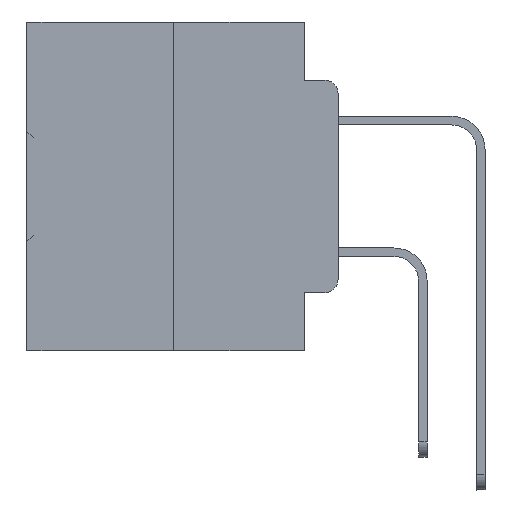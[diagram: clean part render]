
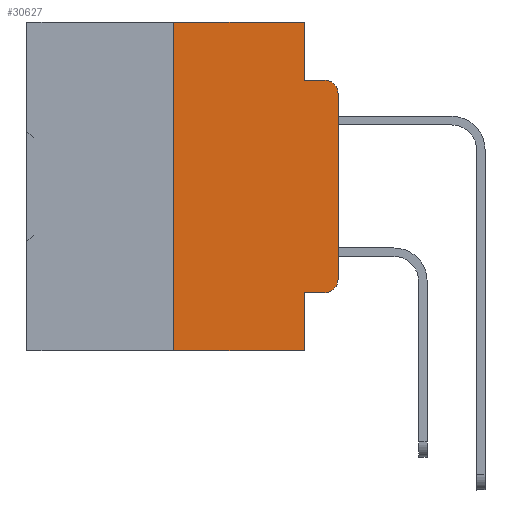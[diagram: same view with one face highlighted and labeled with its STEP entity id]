
A CAD part, left-side view. The second image highlights one B-rep face of the part: STEP entity #30627.
In plain terms, the highlighted planar face has unit normal (-1, 0, 0).
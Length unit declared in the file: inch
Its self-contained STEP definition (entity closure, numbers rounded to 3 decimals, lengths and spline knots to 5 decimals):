
#552 = CARTESIAN_POINT ( 'NONE',  ( 0., 0.25, 0. ) ) ;
#585 = DIRECTION ( 'NONE',  ( 0., 0., -1. ) ) ;
#738 = EDGE_CURVE ( 'NONE', #4777, #22115, #18678, .T. ) ;
#2525 = ORIENTED_EDGE ( 'NONE', *, *, #8999, .T. ) ;
#2659 = VERTEX_POINT ( 'NONE', #24589 ) ;
#2693 = VERTEX_POINT ( 'NONE', #31869 ) ;
#3128 = CARTESIAN_POINT ( 'NONE',  ( 0., 0.051, -0.4115 ) ) ;
#4285 = VERTEX_POINT ( 'NONE', #552 ) ;
#4529 = CARTESIAN_POINT ( 'NONE',  ( 0., 0.051, -0.4115 ) ) ;
#4596 = VECTOR ( 'NONE', #19500, 39.37008 ) ;
#4777 = VERTEX_POINT ( 'NONE', #15202 ) ;
#5955 = VECTOR ( 'NONE', #25425, 39.37008 ) ;
#7775 = CARTESIAN_POINT ( 'NONE',  ( 0., 0., 0. ) ) ;
#8999 = EDGE_CURVE ( 'NONE', #2659, #2693, #24691, .T. ) ;
#9035 = CARTESIAN_POINT ( 'NONE',  ( 0., 0.051, 0. ) ) ;
#11295 = VECTOR ( 'NONE', #35270, 39.37008 ) ;
#12041 = DIRECTION ( 'NONE',  ( 0., 0., -1. ) ) ;
#12151 = EDGE_CURVE ( 'NONE', #31244, #4777, #18021, .T. ) ;
#12279 = DIRECTION ( 'NONE',  ( 0., -1., 0. ) ) ;
#12910 = EDGE_CURVE ( 'NONE', #4285, #19026, #14462, .T. ) ;
#12939 = ORIENTED_EDGE ( 'NONE', *, *, #13993, .F. ) ;
#13425 = EDGE_CURVE ( 'NONE', #21125, #2693, #34283, .T. ) ;
#13529 = LINE ( 'NONE', #4529, #4596 ) ;
#13627 = ORIENTED_EDGE ( 'NONE', *, *, #28277, .T. ) ;
#13688 = CARTESIAN_POINT ( 'NONE',  ( 0., 0.051, -0.0885 ) ) ;
#13993 = EDGE_CURVE ( 'NONE', #19026, #22054, #28721, .T. ) ;
#14462 = LINE ( 'NONE', #29660, #28362 ) ;
#14906 = VECTOR ( 'NONE', #12279, 39.37008 ) ;
#15202 = CARTESIAN_POINT ( 'NONE',  ( 0., 0., -0.1085 ) ) ;
#16266 = DIRECTION ( 'NONE',  ( -1., 0., 0. ) ) ;
#16689 = ORIENTED_EDGE ( 'NONE', *, *, #738, .T. ) ;
#17029 = AXIS2_PLACEMENT_3D ( 'NONE', #24360, #18546, #585 ) ;
#17354 = CARTESIAN_POINT ( 'NONE',  ( 0., 0.051, 0. ) ) ;
#17654 = CARTESIAN_POINT ( 'NONE',  ( 0., 0.051, -0.0885 ) ) ;
#18021 = LINE ( 'NONE', #7775, #31798 ) ;
#18546 = DIRECTION ( 'NONE',  ( 1., 0., 0. ) ) ;
#18632 = EDGE_LOOP ( 'NONE', ( #21597, #16689, #18849, #12939, #20188, #19413, #2525, #19302, #13627, #21815 ) ) ;
#18661 = VECTOR ( 'NONE', #12041, 39.37008 ) ;
#18678 = CIRCLE ( 'NONE', #37210, 0.02 ) ;
#18849 = ORIENTED_EDGE ( 'NONE', *, *, #33315, .F. ) ;
#19026 = VERTEX_POINT ( 'NONE', #17354 ) ;
#19302 = ORIENTED_EDGE ( 'NONE', *, *, #13425, .F. ) ;
#19413 = ORIENTED_EDGE ( 'NONE', *, *, #35477, .F. ) ;
#19500 = DIRECTION ( 'NONE',  ( 0., -1., 0. ) ) ;
#19855 = DIRECTION ( 'NONE',  ( 0., 0., 1. ) ) ;
#19888 = CARTESIAN_POINT ( 'NONE',  ( 0., 0.02, -0.0885 ) ) ;
#20188 = ORIENTED_EDGE ( 'NONE', *, *, #12910, .F. ) ;
#20952 = VECTOR ( 'NONE', #23620, 39.37008 ) ;
#21125 = VERTEX_POINT ( 'NONE', #3128 ) ;
#21597 = ORIENTED_EDGE ( 'NONE', *, *, #12151, .T. ) ;
#21815 = ORIENTED_EDGE ( 'NONE', *, *, #32323, .T. ) ;
#22050 = CARTESIAN_POINT ( 'NONE',  ( 0., 0.02, -0.4115 ) ) ;
#22054 = VERTEX_POINT ( 'NONE', #13688 ) ;
#22115 = VERTEX_POINT ( 'NONE', #19888 ) ;
#22398 = CARTESIAN_POINT ( 'NONE',  ( 0., 0., -0.3915 ) ) ;
#22506 = CARTESIAN_POINT ( 'NONE',  ( 0., 0.25, 0. ) ) ;
#23231 = VERTEX_POINT ( 'NONE', #22050 ) ;
#23620 = DIRECTION ( 'NONE',  ( 0., 0., -1. ) ) ;
#24360 = CARTESIAN_POINT ( 'NONE',  ( 0., 0.473, 0. ) ) ;
#24589 = CARTESIAN_POINT ( 'NONE',  ( 0., 0.25, -0.5 ) ) ;
#24691 = LINE ( 'NONE', #27043, #14906 ) ;
#25425 = DIRECTION ( 'NONE',  ( 0., 0., 1. ) ) ;
#25435 = DIRECTION ( 'NONE',  ( -1., 0., 0. ) ) ;
#27043 = CARTESIAN_POINT ( 'NONE',  ( 0., 0.473, -0.5 ) ) ;
#28277 = EDGE_CURVE ( 'NONE', #21125, #23231, #13529, .T. ) ;
#28362 = VECTOR ( 'NONE', #32626, 39.37008 ) ;
#28599 = FACE_OUTER_BOUND ( 'NONE', #18632, .T. ) ;
#28721 = LINE ( 'NONE', #32295, #20952 ) ;
#29630 = LINE ( 'NONE', #22506, #5955 ) ;
#29660 = CARTESIAN_POINT ( 'NONE',  ( 0., 0.473, 0. ) ) ;
#30627 = ADVANCED_FACE ( 'NONE', ( #28599 ), #36156, .F. ) ;
#31244 = VERTEX_POINT ( 'NONE', #22398 ) ;
#31340 = CIRCLE ( 'NONE', #37045, 0.02 ) ;
#31798 = VECTOR ( 'NONE', #19855, 39.37008 ) ;
#31869 = CARTESIAN_POINT ( 'NONE',  ( 0., 0.051, -0.5 ) ) ;
#32295 = CARTESIAN_POINT ( 'NONE',  ( 0., 0.051, 0. ) ) ;
#32323 = EDGE_CURVE ( 'NONE', #23231, #31244, #31340, .T. ) ;
#32626 = DIRECTION ( 'NONE',  ( 0., -1., 0. ) ) ;
#33315 = EDGE_CURVE ( 'NONE', #22054, #22115, #33961, .T. ) ;
#33908 = CARTESIAN_POINT ( 'NONE',  ( 0., 0.02, -0.3915 ) ) ;
#33961 = LINE ( 'NONE', #17654, #11295 ) ;
#34283 = LINE ( 'NONE', #9035, #18661 ) ;
#35270 = DIRECTION ( 'NONE',  ( 0., -1., 0. ) ) ;
#35477 = EDGE_CURVE ( 'NONE', #2659, #4285, #29630, .T. ) ;
#36156 = PLANE ( 'NONE',  #17029 ) ;
#36697 = CARTESIAN_POINT ( 'NONE',  ( 0., 0.02, -0.1085 ) ) ;
#36886 = DIRECTION ( 'NONE',  ( 0., 0., -1. ) ) ;
#37045 = AXIS2_PLACEMENT_3D ( 'NONE', #33908, #16266, #36886 ) ;
#37210 = AXIS2_PLACEMENT_3D ( 'NONE', #36697, #25435, #37997 ) ;
#37997 = DIRECTION ( 'NONE',  ( 0., 0., -1. ) ) ;
